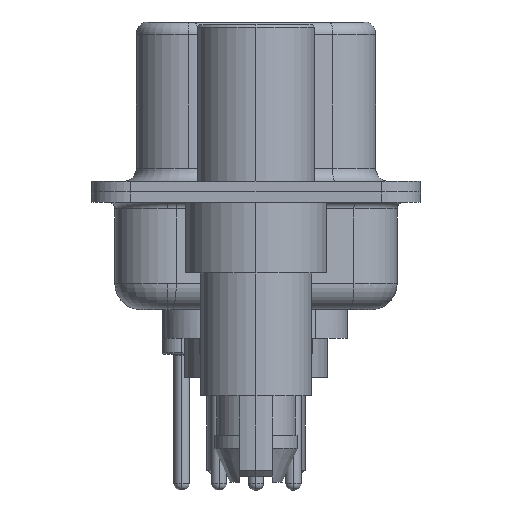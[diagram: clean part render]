
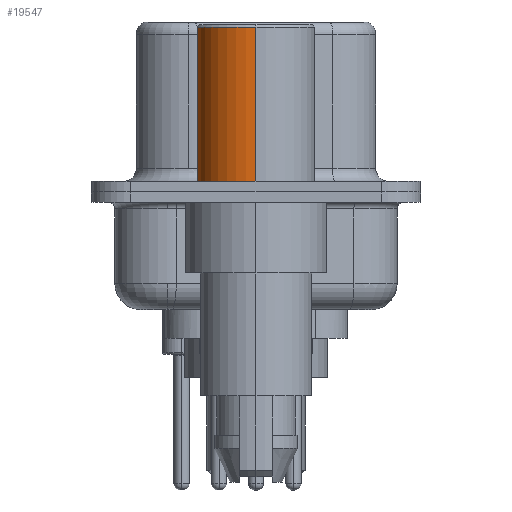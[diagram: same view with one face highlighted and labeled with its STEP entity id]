
A CAD part, left-side view. The second image highlights one B-rep face of the part: STEP entity #19547.
In plain terms, the highlighted cylindrical face has radius 2.25 mm (diameter 4.5 mm), a partial arc.
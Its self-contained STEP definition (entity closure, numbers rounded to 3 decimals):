
#497 = CARTESIAN_POINT ( 'NONE',  ( 0., 0., 0.581 ) ) ;
#1279 = CARTESIAN_POINT ( 'NONE',  ( -2.25, 0., 6.3 ) ) ;
#2366 = LINE ( 'NONE', #4674, #17310 ) ;
#3334 = ORIENTED_EDGE ( 'NONE', *, *, #20417, .T. ) ;
#3762 = DIRECTION ( 'NONE',  ( 1., 0., 0. ) ) ;
#4674 = CARTESIAN_POINT ( 'NONE',  ( 2.25, 0., 0.581 ) ) ;
#4799 = DIRECTION ( 'NONE',  ( 0., 0., 1. ) ) ;
#6254 = CARTESIAN_POINT ( 'NONE',  ( -2.25, 0., 0.4 ) ) ;
#6328 = DIRECTION ( 'NONE',  ( 1., 0., 0. ) ) ;
#6514 = AXIS2_PLACEMENT_3D ( 'NONE', #11326, #4799, #12955 ) ;
#7948 = DIRECTION ( 'NONE',  ( 0., 0., 1. ) ) ;
#8433 = CARTESIAN_POINT ( 'NONE',  ( 2.25, 0., 6.3 ) ) ;
#9028 = CIRCLE ( 'NONE', #19499, 2.25 ) ;
#9892 = ORIENTED_EDGE ( 'NONE', *, *, #18077, .F. ) ;
#10752 = CIRCLE ( 'NONE', #6514, 2.25 ) ;
#10859 = CARTESIAN_POINT ( 'NONE',  ( 2.25, 0., 0.4 ) ) ;
#10980 = ORIENTED_EDGE ( 'NONE', *, *, #19836, .F. ) ;
#11037 = FACE_OUTER_BOUND ( 'NONE', #18437, .T. ) ;
#11299 = CARTESIAN_POINT ( 'NONE',  ( 0., 0., 6.3 ) ) ;
#11326 = CARTESIAN_POINT ( 'NONE',  ( 0., 0., 0.4 ) ) ;
#12848 = DIRECTION ( 'NONE',  ( 0., 0., 1. ) ) ;
#12955 = DIRECTION ( 'NONE',  ( 1., 0., 0. ) ) ;
#14731 = EDGE_CURVE ( 'NONE', #15292, #20306, #14990, .T. ) ;
#14750 = VECTOR ( 'NONE', #18982, 1000. ) ;
#14990 = LINE ( 'NONE', #15469, #14750 ) ;
#15292 = VERTEX_POINT ( 'NONE', #6254 ) ;
#15469 = CARTESIAN_POINT ( 'NONE',  ( -2.25, 0., 0.581 ) ) ;
#16772 = VERTEX_POINT ( 'NONE', #8433 ) ;
#16998 = VERTEX_POINT ( 'NONE', #10859 ) ;
#17310 = VECTOR ( 'NONE', #7948, 1000. ) ;
#17428 = AXIS2_PLACEMENT_3D ( 'NONE', #497, #18111, #3762 ) ;
#18054 = ORIENTED_EDGE ( 'NONE', *, *, #14731, .T. ) ;
#18077 = EDGE_CURVE ( 'NONE', #16772, #20306, #9028, .T. ) ;
#18111 = DIRECTION ( 'NONE',  ( 0., 0., 1. ) ) ;
#18437 = EDGE_LOOP ( 'NONE', ( #3334, #18054, #9892, #10980 ) ) ;
#18982 = DIRECTION ( 'NONE',  ( 0., 0., 1. ) ) ;
#19107 = CYLINDRICAL_SURFACE ( 'NONE', #17428, 2.25 ) ;
#19499 = AXIS2_PLACEMENT_3D ( 'NONE', #11299, #12848, #6328 ) ;
#19547 = ADVANCED_FACE ( 'NONE', ( #11037 ), #19107, .T. ) ;
#19836 = EDGE_CURVE ( 'NONE', #16998, #16772, #2366, .T. ) ;
#20306 = VERTEX_POINT ( 'NONE', #1279 ) ;
#20417 = EDGE_CURVE ( 'NONE', #16998, #15292, #10752, .T. ) ;
